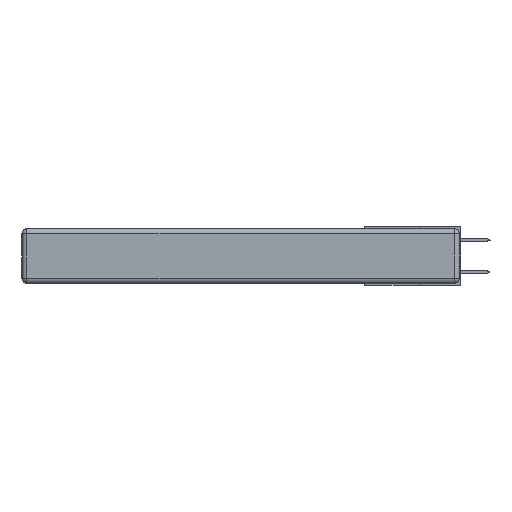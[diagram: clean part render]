
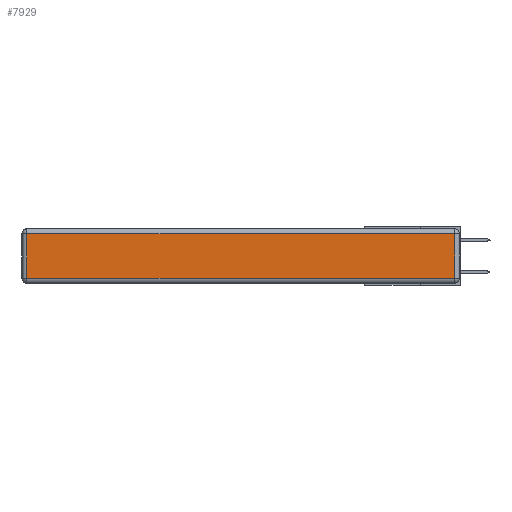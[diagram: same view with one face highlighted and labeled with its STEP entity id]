
A CAD part, left-side view. The second image highlights one B-rep face of the part: STEP entity #7929.
In plain terms, the highlighted planar face has unit normal (-1, 0, 0).
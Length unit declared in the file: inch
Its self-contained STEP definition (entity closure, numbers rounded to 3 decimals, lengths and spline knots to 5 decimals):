
#1233 = CARTESIAN_POINT ( 'NONE',  ( 0., 0.03, -0.343 ) ) ;
#1658 = VERTEX_POINT ( 'NONE', #11920 ) ;
#2122 = ORIENTED_EDGE ( 'NONE', *, *, #17180, .T. ) ;
#2645 = EDGE_CURVE ( 'NONE', #1658, #13905, #11665, .T. ) ;
#2736 = EDGE_CURVE ( 'NONE', #13905, #4236, #18425, .T. ) ;
#3289 = AXIS2_PLACEMENT_3D ( 'NONE', #13553, #15109, #5878 ) ;
#3835 = ORIENTED_EDGE ( 'NONE', *, *, #8489, .T. ) ;
#3994 = CARTESIAN_POINT ( 'NONE',  ( 0., 2.75, -0.03 ) ) ;
#4236 = VERTEX_POINT ( 'NONE', #4285 ) ;
#4285 = CARTESIAN_POINT ( 'NONE',  ( 0., 0.03, -0.313 ) ) ;
#5878 = DIRECTION ( 'NONE',  ( 0., 0., 1. ) ) ;
#6011 = DIRECTION ( 'NONE',  ( 0., 0., -1. ) ) ;
#7929 = ADVANCED_FACE ( 'NONE', ( #17762 ), #8946, .T. ) ;
#8241 = LINE ( 'NONE', #1233, #19796 ) ;
#8489 = EDGE_CURVE ( 'NONE', #10952, #1658, #19947, .T. ) ;
#8946 = PLANE ( 'NONE',  #3289 ) ;
#10285 = DIRECTION ( 'NONE',  ( 0., 1., 0. ) ) ;
#10728 = VECTOR ( 'NONE', #12350, 39.37008 ) ;
#10811 = CARTESIAN_POINT ( 'NONE',  ( 0., 0., -0.313 ) ) ;
#10952 = VERTEX_POINT ( 'NONE', #13504 ) ;
#11665 = LINE ( 'NONE', #12283, #18892 ) ;
#11920 = CARTESIAN_POINT ( 'NONE',  ( 0., 2.72, -0.03 ) ) ;
#12036 = DIRECTION ( 'NONE',  ( 0., 0., 1. ) ) ;
#12283 = CARTESIAN_POINT ( 'NONE',  ( 0., 2.72, -0.343 ) ) ;
#12350 = DIRECTION ( 'NONE',  ( 0., -1., 0. ) ) ;
#13391 = ORIENTED_EDGE ( 'NONE', *, *, #2645, .T. ) ;
#13504 = CARTESIAN_POINT ( 'NONE',  ( 0., 0.03, -0.03 ) ) ;
#13549 = EDGE_LOOP ( 'NONE', ( #18722, #2122, #3835, #13391 ) ) ;
#13553 = CARTESIAN_POINT ( 'NONE',  ( 0., 0., -0.343 ) ) ;
#13905 = VERTEX_POINT ( 'NONE', #18375 ) ;
#14145 = VECTOR ( 'NONE', #10285, 39.37008 ) ;
#15109 = DIRECTION ( 'NONE',  ( -1., 0., 0. ) ) ;
#17180 = EDGE_CURVE ( 'NONE', #4236, #10952, #8241, .T. ) ;
#17762 = FACE_OUTER_BOUND ( 'NONE', #13549, .T. ) ;
#18375 = CARTESIAN_POINT ( 'NONE',  ( 0., 2.72, -0.313 ) ) ;
#18425 = LINE ( 'NONE', #10811, #10728 ) ;
#18722 = ORIENTED_EDGE ( 'NONE', *, *, #2736, .T. ) ;
#18892 = VECTOR ( 'NONE', #6011, 39.37008 ) ;
#19796 = VECTOR ( 'NONE', #12036, 39.37008 ) ;
#19947 = LINE ( 'NONE', #3994, #14145 ) ;
